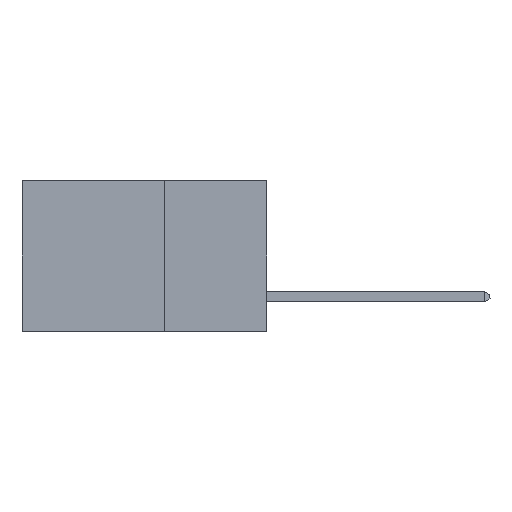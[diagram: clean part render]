
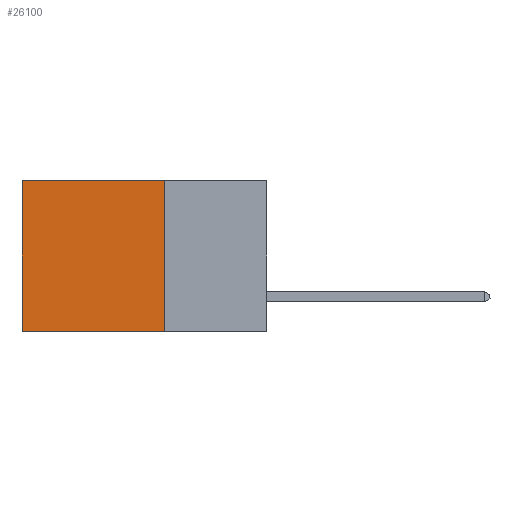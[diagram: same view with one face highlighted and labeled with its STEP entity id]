
A CAD part, left-side view. The second image highlights one B-rep face of the part: STEP entity #26100.
In plain terms, the highlighted planar face has unit normal (-1, 0, 0).
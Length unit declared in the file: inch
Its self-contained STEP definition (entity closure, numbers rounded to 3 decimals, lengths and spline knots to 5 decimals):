
#554 = ORIENTED_EDGE ( 'NONE', *, *, #4539, .T. ) ;
#806 = EDGE_LOOP ( 'NONE', ( #554, #13243, #2293, #17272 ) ) ;
#947 = LINE ( 'NONE', #23187, #27989 ) ;
#2293 = ORIENTED_EDGE ( 'NONE', *, *, #7403, .F. ) ;
#2530 = CARTESIAN_POINT ( 'NONE',  ( 0.2875, 0.25, -0.37 ) ) ;
#2814 = EDGE_CURVE ( 'NONE', #16548, #30240, #15430, .T. ) ;
#3550 = CARTESIAN_POINT ( 'NONE',  ( 0.2875, 0.25, 0. ) ) ;
#3854 = DIRECTION ( 'NONE',  ( 0., 0., -1. ) ) ;
#4539 = EDGE_CURVE ( 'NONE', #11286, #30240, #22782, .T. ) ;
#5731 = EDGE_CURVE ( 'NONE', #12224, #11286, #5909, .T. ) ;
#5909 = LINE ( 'NONE', #3550, #6724 ) ;
#6724 = VECTOR ( 'NONE', #21344, 39.37008 ) ;
#7403 = EDGE_CURVE ( 'NONE', #12224, #16548, #947, .T. ) ;
#7977 = DIRECTION ( 'NONE',  ( 0., 0., -1. ) ) ;
#8087 = CARTESIAN_POINT ( 'NONE',  ( 0.2875, 0.25, 0. ) ) ;
#8096 = CARTESIAN_POINT ( 'NONE',  ( 0.2875, 0.6, -0.37 ) ) ;
#10666 = DIRECTION ( 'NONE',  ( 1., 0., 0. ) ) ;
#11286 = VERTEX_POINT ( 'NONE', #15291 ) ;
#12224 = VERTEX_POINT ( 'NONE', #31518 ) ;
#13243 = ORIENTED_EDGE ( 'NONE', *, *, #2814, .F. ) ;
#13548 = FACE_OUTER_BOUND ( 'NONE', #806, .T. ) ;
#14623 = VECTOR ( 'NONE', #27967, 39.37008 ) ;
#15291 = CARTESIAN_POINT ( 'NONE',  ( 0.2875, 0.6, 0. ) ) ;
#15430 = LINE ( 'NONE', #2530, #14623 ) ;
#16092 = VECTOR ( 'NONE', #3854, 39.37008 ) ;
#16548 = VERTEX_POINT ( 'NONE', #18255 ) ;
#17272 = ORIENTED_EDGE ( 'NONE', *, *, #5731, .T. ) ;
#17630 = AXIS2_PLACEMENT_3D ( 'NONE', #8087, #10666, #28350 ) ;
#18255 = CARTESIAN_POINT ( 'NONE',  ( 0.2875, 0.25, -0.37 ) ) ;
#21344 = DIRECTION ( 'NONE',  ( 0., 1., 0. ) ) ;
#22782 = LINE ( 'NONE', #29267, #16092 ) ;
#23187 = CARTESIAN_POINT ( 'NONE',  ( 0.2875, 0.25, 0. ) ) ;
#25826 = PLANE ( 'NONE',  #17630 ) ;
#26100 = ADVANCED_FACE ( 'NONE', ( #13548 ), #25826, .F. ) ;
#27967 = DIRECTION ( 'NONE',  ( 0., 1., 0. ) ) ;
#27989 = VECTOR ( 'NONE', #7977, 39.37008 ) ;
#28350 = DIRECTION ( 'NONE',  ( 0., 0., -1. ) ) ;
#29267 = CARTESIAN_POINT ( 'NONE',  ( 0.2875, 0.6, 0. ) ) ;
#30240 = VERTEX_POINT ( 'NONE', #8096 ) ;
#31518 = CARTESIAN_POINT ( 'NONE',  ( 0.2875, 0.25, 0. ) ) ;
